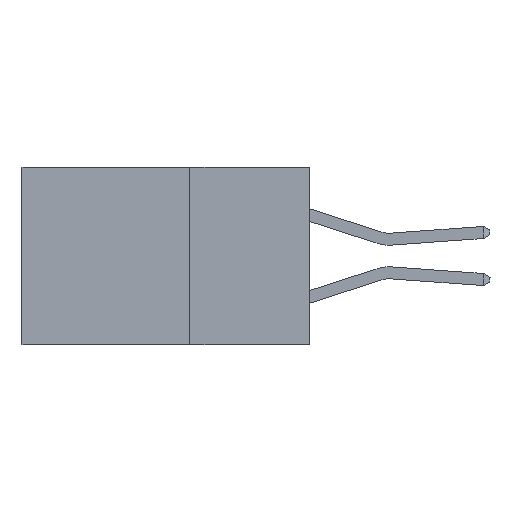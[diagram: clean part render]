
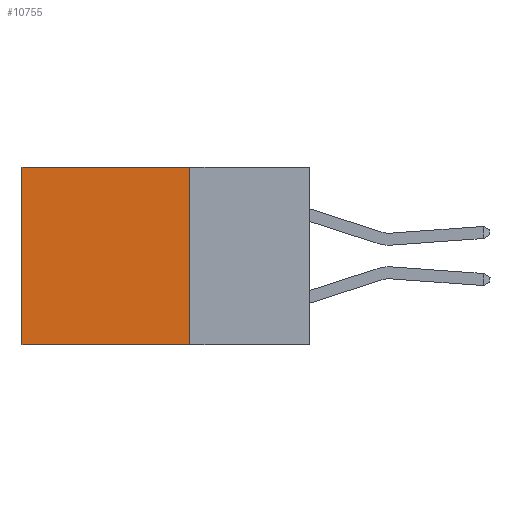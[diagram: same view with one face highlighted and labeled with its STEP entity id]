
A CAD part, left-side view. The second image highlights one B-rep face of the part: STEP entity #10755.
In plain terms, the highlighted planar face has unit normal (-1, 0, 0).
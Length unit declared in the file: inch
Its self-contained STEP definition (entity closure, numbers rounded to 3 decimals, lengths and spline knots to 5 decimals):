
#540 = LINE ( 'NONE', #15971, #13540 ) ;
#841 = DIRECTION ( 'NONE',  ( 0., 0., -1. ) ) ;
#948 = DIRECTION ( 'NONE',  ( 1., 0., 0. ) ) ;
#1847 = ORIENTED_EDGE ( 'NONE', *, *, #7838, .T. ) ;
#2533 = VERTEX_POINT ( 'NONE', #4870 ) ;
#3328 = EDGE_CURVE ( 'NONE', #7581, #7208, #18476, .T. ) ;
#4870 = CARTESIAN_POINT ( 'NONE',  ( 0.2615, 0.6, 0. ) ) ;
#6025 = VERTEX_POINT ( 'NONE', #19484 ) ;
#7191 = CARTESIAN_POINT ( 'NONE',  ( 0.2615, 0.6, -0.37 ) ) ;
#7208 = VERTEX_POINT ( 'NONE', #7191 ) ;
#7228 = ORIENTED_EDGE ( 'NONE', *, *, #13581, .T. ) ;
#7581 = VERTEX_POINT ( 'NONE', #8120 ) ;
#7609 = VECTOR ( 'NONE', #15483, 39.37008 ) ;
#7838 = EDGE_CURVE ( 'NONE', #6025, #2533, #8135, .T. ) ;
#8120 = CARTESIAN_POINT ( 'NONE',  ( 0.2615, 0.25, -0.37 ) ) ;
#8135 = LINE ( 'NONE', #20281, #7609 ) ;
#10015 = EDGE_CURVE ( 'NONE', #6025, #7581, #540, .T. ) ;
#10198 = LINE ( 'NONE', #11494, #13077 ) ;
#10755 = ADVANCED_FACE ( 'NONE', ( #16360 ), #11148, .F. ) ;
#10757 = VECTOR ( 'NONE', #14275, 39.37008 ) ;
#11148 = PLANE ( 'NONE',  #21450 ) ;
#11494 = CARTESIAN_POINT ( 'NONE',  ( 0.2615, 0.6, -0.37 ) ) ;
#11918 = EDGE_LOOP ( 'NONE', ( #7228, #12660, #15398, #1847 ) ) ;
#12660 = ORIENTED_EDGE ( 'NONE', *, *, #3328, .F. ) ;
#12852 = DIRECTION ( 'NONE',  ( 0., 0., -1. ) ) ;
#13077 = VECTOR ( 'NONE', #13257, 39.37008 ) ;
#13257 = DIRECTION ( 'NONE',  ( 0., 0., -1. ) ) ;
#13540 = VECTOR ( 'NONE', #841, 39.37008 ) ;
#13581 = EDGE_CURVE ( 'NONE', #2533, #7208, #10198, .T. ) ;
#14275 = DIRECTION ( 'NONE',  ( 0., 1., 0. ) ) ;
#15398 = ORIENTED_EDGE ( 'NONE', *, *, #10015, .F. ) ;
#15483 = DIRECTION ( 'NONE',  ( 0., 1., 0. ) ) ;
#15971 = CARTESIAN_POINT ( 'NONE',  ( 0.2615, 0.25, -0.37 ) ) ;
#16360 = FACE_OUTER_BOUND ( 'NONE', #11918, .T. ) ;
#18476 = LINE ( 'NONE', #18971, #10757 ) ;
#18971 = CARTESIAN_POINT ( 'NONE',  ( 0.2615, 0.25, -0.37 ) ) ;
#19484 = CARTESIAN_POINT ( 'NONE',  ( 0.2615, 0.25, 0. ) ) ;
#20281 = CARTESIAN_POINT ( 'NONE',  ( 0.2615, 0.25, 0. ) ) ;
#20950 = CARTESIAN_POINT ( 'NONE',  ( 0.2615, 0.25, -0.37 ) ) ;
#21450 = AXIS2_PLACEMENT_3D ( 'NONE', #20950, #948, #12852 ) ;
